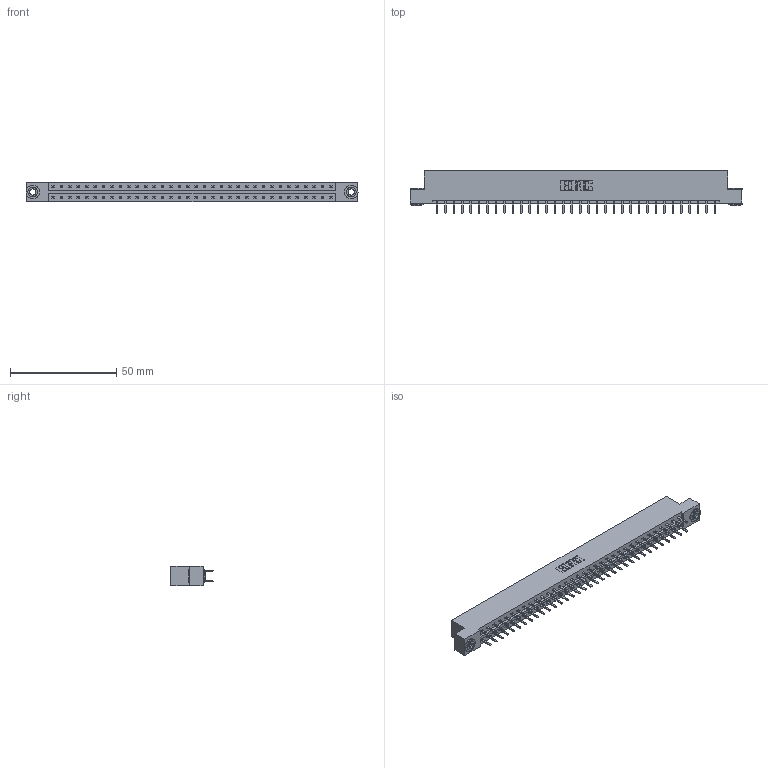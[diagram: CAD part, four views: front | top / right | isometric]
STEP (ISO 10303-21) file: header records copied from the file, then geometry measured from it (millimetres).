
FILE_DESCRIPTION (( 'STEP AP203' ), '1' );
FILE_NAME ('833-068-520-203.STEP', '2020-06-05T10:03:56', ( '' ), ( '' ), 'SwSTEP 2.0', 'SolidWorks 2020', '' );
FILE_SCHEMA (( 'CONFIG_CONTROL_DESIGN' ));
Length unit declared in the file: inch
Products named in the file (4): 833-068-520-203; 345-250-002_345-250-002-102; 833 Part_Flush - .156 Dia - TH; 345-292-001_345-293-120
Assembly tree (71 placements, depth 2):
  833-068-520-203
    833 Part_Flush - .156 Dia - TH
    345-292-001_345-293-120  x68
    345-250-002_345-250-002-102  x2
Bounding box: 156.26 x 20.02 x 9.4 mm (x, y, z)
Volume: 15868 mm3; surface area: 18815.7 mm2
Topology: 71 solids, 71 shells, 3960 faces, 11471 edges, 7462 vertices
Faces by surface type: plane 2664, cylinder 1288, cone 8
Entity records: 23672 total; most frequent: CARTESIAN_POINT 3921, ORIENTED_EDGE 3838, DIRECTION 3385, EDGE_CURVE 1919, VECTOR 1763, LINE 1763, VERTEX_POINT 1274, AXIS2_PLACEMENT_3D 811
